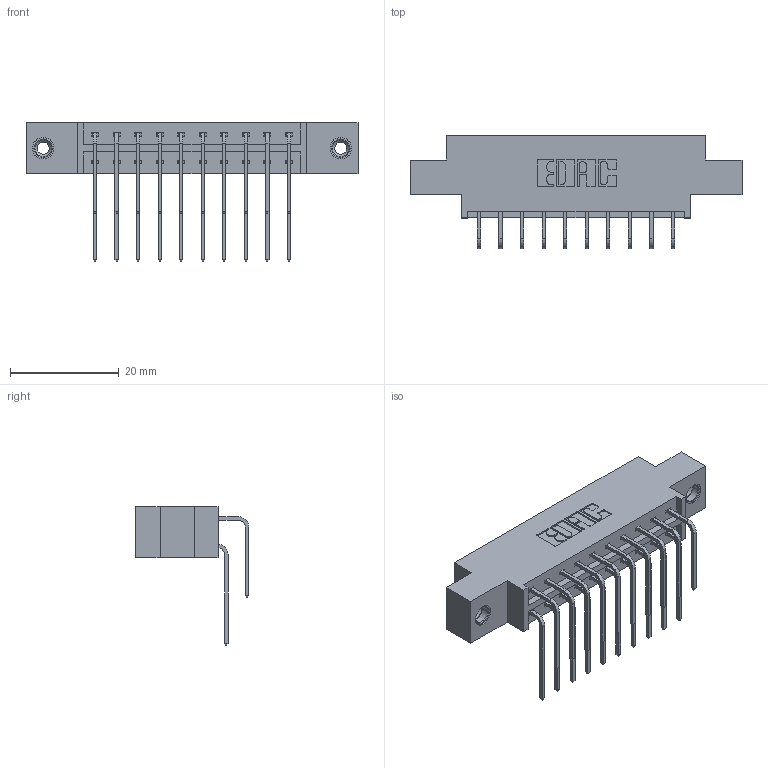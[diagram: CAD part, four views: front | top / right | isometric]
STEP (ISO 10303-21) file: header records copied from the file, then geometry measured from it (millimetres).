
FILE_DESCRIPTION (( 'STEP AP203' ), '1' );
FILE_NAME ('833-020-559-808.STEP', '2020-06-01T14:17:23', ( '' ), ( '' ), 'SwSTEP 2.0', 'SolidWorks 2020', '' );
FILE_SCHEMA (( 'CONFIG_CONTROL_DESIGN' ));
Length unit declared in the file: inch
Products named in the file (5): 345-292-001_559 Tail - 2; 345-250-001_345-250-003-102; 833-020-559-808; 345-292-001_558 559 Tail - 1; 833 Part_Offset - .156 Dia - TI
Assembly tree (23 placements, depth 2):
  833-020-559-808
    833 Part_Offset - .156 Dia - TI
    345-292-001_558 559 Tail - 1  x10
    345-292-001_559 Tail - 2  x10
    345-250-001_345-250-003-102  x2
Bounding box: 61.16 x 20.9 x 25.53 mm (x, y, z)
Volume: 5826.2 mm3; surface area: 7361.5 mm2
Topology: 23 solids, 23 shells, 1258 faces, 3679 edges, 2418 vertices
Faces by surface type: plane 866, cylinder 376, cone 12, torus 4
Entity records: 13674 total; most frequent: CARTESIAN_POINT 2340, ORIENTED_EDGE 2218, DIRECTION 2067, EDGE_CURVE 1109, VECTOR 921, LINE 921, VERTEX_POINT 732, AXIS2_PLACEMENT_3D 573
